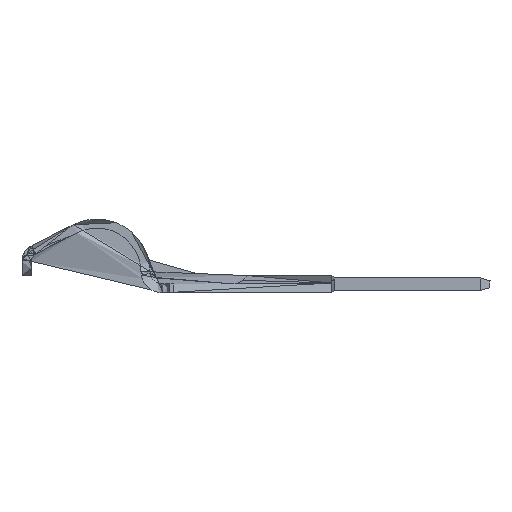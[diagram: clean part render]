
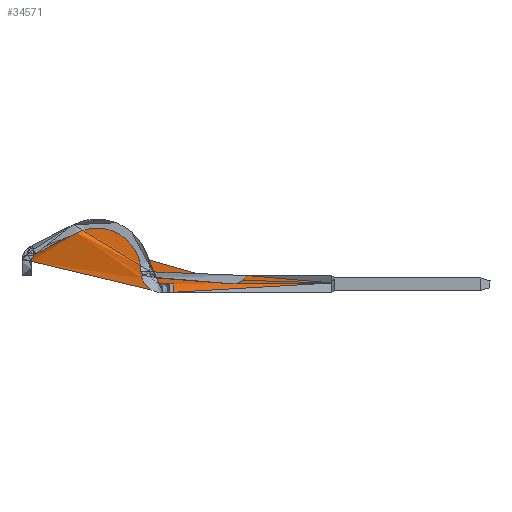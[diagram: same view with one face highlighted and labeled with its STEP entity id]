
A CAD part, left-side view. The second image highlights one B-rep face of the part: STEP entity #34571.
In plain terms, the highlighted face is planar.
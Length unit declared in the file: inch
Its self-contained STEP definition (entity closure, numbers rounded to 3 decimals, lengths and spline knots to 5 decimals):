
#806 = LINE ( 'NONE', #4842, #37868 ) ;
#927 = CARTESIAN_POINT ( 'NONE',  ( 0.14622, 0.058, -0.025 ) ) ;
#1378 = ORIENTED_EDGE ( 'NONE', *, *, #48905, .F. ) ;
#1527 = VECTOR ( 'NONE', #22782, 39.37008 ) ;
#2349 = VERTEX_POINT ( 'NONE', #21564 ) ;
#3580 = CARTESIAN_POINT ( 'NONE',  ( 0.33619, 0.044, -0.025 ) ) ;
#3654 = DIRECTION ( 'NONE',  ( 0.893, 0.449, 0. ) ) ;
#3703 = LINE ( 'NONE', #7506, #1527 ) ;
#3795 = ORIENTED_EDGE ( 'NONE', *, *, #23515, .T. ) ;
#4460 = EDGE_CURVE ( 'NONE', #13164, #30837, #806, .T. ) ;
#4842 = CARTESIAN_POINT ( 'NONE',  ( 0.15365, 0.06956, -0.025 ) ) ;
#6113 = CARTESIAN_POINT ( 'NONE',  ( 0.58021, 0.0125, -0.025 ) ) ;
#6319 = ORIENTED_EDGE ( 'NONE', *, *, #16353, .F. ) ;
#6329 = CARTESIAN_POINT ( 'NONE',  ( 0.15971, 0.0575, -0.025 ) ) ;
#6634 = VERTEX_POINT ( 'NONE', #22959 ) ;
#6862 = CARTESIAN_POINT ( 'NONE',  ( 0.45821, 0.0375, -0.025 ) ) ;
#7190 = ORIENTED_EDGE ( 'NONE', *, *, #17108, .F. ) ;
#7205 = CIRCLE ( 'NONE', #41186, 0.02173 ) ;
#7506 = CARTESIAN_POINT ( 'NONE',  ( 0.33619, 0.0125, -0.025 ) ) ;
#11875 = PLANE ( 'NONE',  #24773 ) ;
#12076 = VERTEX_POINT ( 'NONE', #927 ) ;
#12483 = ORIENTED_EDGE ( 'NONE', *, *, #4460, .F. ) ;
#13052 = VECTOR ( 'NONE', #28300, 39.37008 ) ;
#13164 = VERTEX_POINT ( 'NONE', #19056 ) ;
#13647 = CARTESIAN_POINT ( 'NONE',  ( 0.2412, 0.0425, -0.025 ) ) ;
#14194 = DIRECTION ( 'NONE',  ( 0., 0., 1. ) ) ;
#14227 = DIRECTION ( 'NONE',  ( 0., 0., -1. ) ) ;
#14764 = LINE ( 'NONE', #6862, #41487 ) ;
#15117 = VERTEX_POINT ( 'NONE', #47750 ) ;
#16353 = EDGE_CURVE ( 'NONE', #15117, #30049, #46870, .T. ) ;
#16976 = VERTEX_POINT ( 'NONE', #20277 ) ;
#17108 = EDGE_CURVE ( 'NONE', #30837, #15117, #41217, .T. ) ;
#17753 = CARTESIAN_POINT ( 'NONE',  ( 0.33619, 0.044, -0.025 ) ) ;
#17786 = CARTESIAN_POINT ( 'NONE',  ( 0.45258, 0.03186, -0.025 ) ) ;
#18234 = LINE ( 'NONE', #22051, #43056 ) ;
#19056 = CARTESIAN_POINT ( 'NONE',  ( 0.15365, 0.06956, -0.025 ) ) ;
#20277 = CARTESIAN_POINT ( 'NONE',  ( 0.31769, 0.04371, -0.025 ) ) ;
#21485 = EDGE_CURVE ( 'NONE', #12076, #2349, #18234, .T. ) ;
#21564 = CARTESIAN_POINT ( 'NONE',  ( 0.13322, 0.058, -0.025 ) ) ;
#22051 = CARTESIAN_POINT ( 'NONE',  ( 0.13321, 0.058, -0.025 ) ) ;
#22782 = DIRECTION ( 'NONE',  ( 1., 0., 0. ) ) ;
#22959 = CARTESIAN_POINT ( 'NONE',  ( 0.33619, 0.0255, -0.025 ) ) ;
#23515 = EDGE_CURVE ( 'NONE', #30199, #38693, #48108, .T. ) ;
#24155 = EDGE_CURVE ( 'NONE', #27555, #30199, #14764, .T. ) ;
#24773 = AXIS2_PLACEMENT_3D ( 'NONE', #28117, #31930, #47189 ) ;
#25321 = DIRECTION ( 'NONE',  ( 0., 0., -1. ) ) ;
#26194 = DIRECTION ( 'NONE',  ( 0.707, 0.707, 0. ) ) ;
#26580 = DIRECTION ( 'NONE',  ( 0., 0., 1. ) ) ;
#27555 = VERTEX_POINT ( 'NONE', #17786 ) ;
#27571 = EDGE_CURVE ( 'NONE', #2349, #41000, #43469, .T. ) ;
#27626 = FACE_OUTER_BOUND ( 'NONE', #30922, .T. ) ;
#28117 = CARTESIAN_POINT ( 'NONE',  ( 0.095, 0.025, -0.025 ) ) ;
#28300 = DIRECTION ( 'NONE',  ( 1., 0., 0. ) ) ;
#29411 = ORIENTED_EDGE ( 'NONE', *, *, #21485, .T. ) ;
#29681 = DIRECTION ( 'NONE',  ( 1., 0., 0. ) ) ;
#29710 = DIRECTION ( 'NONE',  ( -1., 0., 0. ) ) ;
#30049 = VERTEX_POINT ( 'NONE', #49763 ) ;
#30199 = VERTEX_POINT ( 'NONE', #32416 ) ;
#30454 = ORIENTED_EDGE ( 'NONE', *, *, #27571, .T. ) ;
#30837 = VERTEX_POINT ( 'NONE', #40486 ) ;
#30922 = EDGE_LOOP ( 'NONE', ( #18446744073709551615, #29411, #30454, #18446744073709551615, #18446744073709551615, #46974, #18446744073709551615, #32390, #43660, #3795, #18446744073709551615, #1378, #6319, #7190, #12483 ) ) ;
#31252 = DIRECTION ( 'NONE',  ( 1., 0., 0. ) ) ;
#31930 = DIRECTION ( 'NONE',  ( 0., 0., 1. ) ) ;
#32390 = ORIENTED_EDGE ( 'NONE', *, *, #47585, .T. ) ;
#32416 = CARTESIAN_POINT ( 'NONE',  ( 0.45821, 0.0375, -0.025 ) ) ;
#33209 = VERTEX_POINT ( 'NONE', #46195 ) ;
#33434 = DIRECTION ( 'NONE',  ( -1., 0., 0. ) ) ;
#34571 = ADVANCED_FACE ( 'NONE', ( #27626 ), #11875, .F. ) ;
#34597 = AXIS2_PLACEMENT_3D ( 'NONE', #13647, #25321, #33434 ) ;
#35918 = CARTESIAN_POINT ( 'NONE',  ( 0.45821, 0.0375, -0.025 ) ) ;
#36562 = CARTESIAN_POINT ( 'NONE',  ( 0.14781, 0.08118, -0.025 ) ) ;
#37868 = VECTOR ( 'NONE', #3654, 39.37008 ) ;
#37994 = CIRCLE ( 'NONE', #38838, 0.0185 ) ;
#38252 = CARTESIAN_POINT ( 'NONE',  ( 0.43721, 0.04723, -0.025 ) ) ;
#38626 = DIRECTION ( 'NONE',  ( 0., 0., 1. ) ) ;
#38693 = VERTEX_POINT ( 'NONE', #39012 ) ;
#38838 = AXIS2_PLACEMENT_3D ( 'NONE', #17753, #14194, #29681 ) ;
#39012 = CARTESIAN_POINT ( 'NONE',  ( 0.58021, 0.0375, -0.025 ) ) ;
#39403 = AXIS2_PLACEMENT_3D ( 'NONE', #6329, #14227, #29710 ) ;
#40486 = CARTESIAN_POINT ( 'NONE',  ( 0.21268, 0.09924, -0.025 ) ) ;
#41000 = VERTEX_POINT ( 'NONE', #36562 ) ;
#41186 = AXIS2_PLACEMENT_3D ( 'NONE', #38252, #26580, #49454 ) ;
#41217 = CIRCLE ( 'NONE', #34597, 0.0635 ) ;
#41487 = VECTOR ( 'NONE', #26194, 39.37008 ) ;
#43056 = VECTOR ( 'NONE', #48721, 39.37008 ) ;
#43469 = CIRCLE ( 'NONE', #39403, 0.0265 ) ;
#43660 = ORIENTED_EDGE ( 'NONE', *, *, #24155, .T. ) ;
#46195 = CARTESIAN_POINT ( 'NONE',  ( 0.43721, 0.0255, -0.025 ) ) ;
#46870 = CIRCLE ( 'NONE', #48499, 0.0315 ) ;
#46974 = ORIENTED_EDGE ( 'NONE', *, *, #47098, .T. ) ;
#47098 = EDGE_CURVE ( 'NONE', #16976, #6634, #37994, .T. ) ;
#47189 = DIRECTION ( 'NONE',  ( 1., 0., 0. ) ) ;
#47585 = EDGE_CURVE ( 'NONE', #33209, #27555, #7205, .T. ) ;
#47750 = CARTESIAN_POINT ( 'NONE',  ( 0.30469, 0.0435, -0.025 ) ) ;
#48108 = LINE ( 'NONE', #35918, #13052 ) ;
#48467 = VERTEX_POINT ( 'NONE', #6113 ) ;
#48499 = AXIS2_PLACEMENT_3D ( 'NONE', #3580, #38626, #31252 ) ;
#48721 = DIRECTION ( 'NONE',  ( -1., 0., 0. ) ) ;
#48905 = EDGE_CURVE ( 'NONE', #30049, #48467, #3703, .T. ) ;
#49454 = DIRECTION ( 'NONE',  ( 1., 0., 0. ) ) ;
#49763 = CARTESIAN_POINT ( 'NONE',  ( 0.33619, 0.0125, -0.025 ) ) ;
